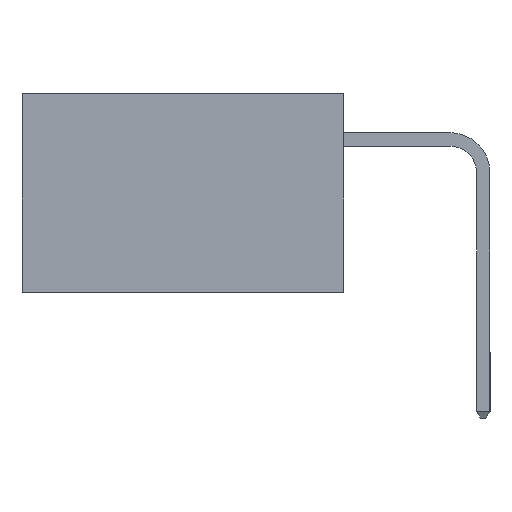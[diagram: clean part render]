
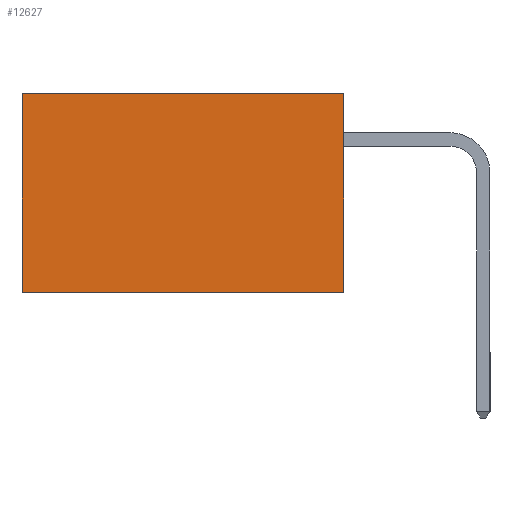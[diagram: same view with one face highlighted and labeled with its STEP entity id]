
A CAD part, left-side view. The second image highlights one B-rep face of the part: STEP entity #12627.
In plain terms, the highlighted planar face has unit normal (-1, 0, 0).
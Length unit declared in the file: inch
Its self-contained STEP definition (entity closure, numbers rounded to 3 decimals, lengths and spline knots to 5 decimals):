
#72 = CARTESIAN_POINT ( 'NONE',  ( 0.2615, 0., -0.37 ) ) ;
#201 = LINE ( 'NONE', #12418, #14179 ) ;
#943 = DIRECTION ( 'NONE',  ( 0., 1., 0. ) ) ;
#1018 = EDGE_LOOP ( 'NONE', ( #7946, #2813, #4282, #10431 ) ) ;
#1071 = CARTESIAN_POINT ( 'NONE',  ( 0.2615, 0., -0.37 ) ) ;
#1448 = VERTEX_POINT ( 'NONE', #1576 ) ;
#1518 = AXIS2_PLACEMENT_3D ( 'NONE', #5684, #4311, #2358 ) ;
#1576 = CARTESIAN_POINT ( 'NONE',  ( 0.2615, 0., 0. ) ) ;
#2237 = DIRECTION ( 'NONE',  ( 0., 1., 0. ) ) ;
#2358 = DIRECTION ( 'NONE',  ( 0., 0., -1. ) ) ;
#2789 = VERTEX_POINT ( 'NONE', #11256 ) ;
#2813 = ORIENTED_EDGE ( 'NONE', *, *, #8280, .F. ) ;
#3355 = CARTESIAN_POINT ( 'NONE',  ( 0.2615, 0.6, -0.37 ) ) ;
#3580 = EDGE_CURVE ( 'NONE', #2789, #5582, #10923, .T. ) ;
#3887 = VECTOR ( 'NONE', #2237, 39.37008 ) ;
#4282 = ORIENTED_EDGE ( 'NONE', *, *, #7910, .F. ) ;
#4311 = DIRECTION ( 'NONE',  ( 1., 0., 0. ) ) ;
#4803 = VECTOR ( 'NONE', #12150, 39.37008 ) ;
#4814 = VECTOR ( 'NONE', #943, 39.37008 ) ;
#5582 = VERTEX_POINT ( 'NONE', #6879 ) ;
#5684 = CARTESIAN_POINT ( 'NONE',  ( 0.2615, 0., -0.37 ) ) ;
#6714 = FACE_OUTER_BOUND ( 'NONE', #1018, .T. ) ;
#6879 = CARTESIAN_POINT ( 'NONE',  ( 0.2615, 0.6, -0.37 ) ) ;
#7910 = EDGE_CURVE ( 'NONE', #1448, #9773, #201, .T. ) ;
#7946 = ORIENTED_EDGE ( 'NONE', *, *, #3580, .T. ) ;
#8099 = EDGE_CURVE ( 'NONE', #1448, #2789, #12860, .T. ) ;
#8280 = EDGE_CURVE ( 'NONE', #9773, #5582, #10063, .T. ) ;
#9773 = VERTEX_POINT ( 'NONE', #72 ) ;
#10063 = LINE ( 'NONE', #1071, #3887 ) ;
#10431 = ORIENTED_EDGE ( 'NONE', *, *, #8099, .T. ) ;
#10888 = CARTESIAN_POINT ( 'NONE',  ( 0.2615, 0., 0. ) ) ;
#10923 = LINE ( 'NONE', #3355, #4803 ) ;
#11256 = CARTESIAN_POINT ( 'NONE',  ( 0.2615, 0.6, 0. ) ) ;
#11283 = PLANE ( 'NONE',  #1518 ) ;
#12150 = DIRECTION ( 'NONE',  ( 0., 0., -1. ) ) ;
#12418 = CARTESIAN_POINT ( 'NONE',  ( 0.2615, 0., -0.37 ) ) ;
#12627 = ADVANCED_FACE ( 'NONE', ( #6714 ), #11283, .F. ) ;
#12860 = LINE ( 'NONE', #10888, #4814 ) ;
#13599 = DIRECTION ( 'NONE',  ( 0., 0., -1. ) ) ;
#14179 = VECTOR ( 'NONE', #13599, 39.37008 ) ;
